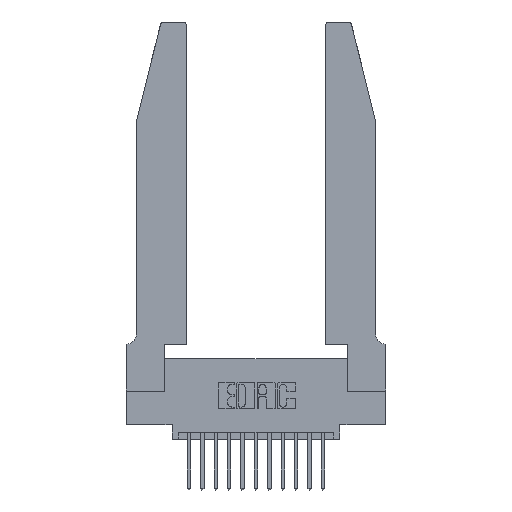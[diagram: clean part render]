
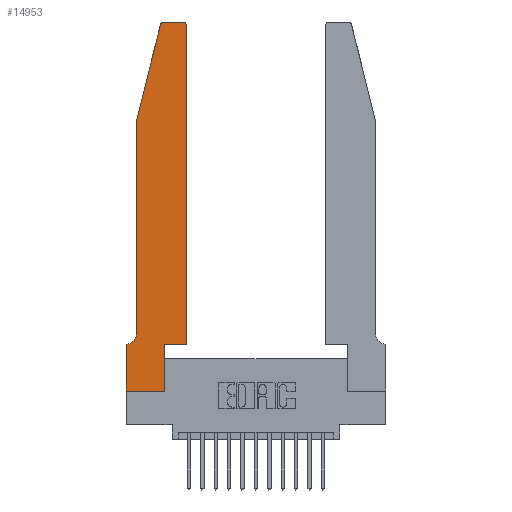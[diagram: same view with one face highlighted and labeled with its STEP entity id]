
A CAD part, top view. The second image highlights one B-rep face of the part: STEP entity #14953.
In plain terms, the highlighted planar face has unit normal (0, 0, 1).
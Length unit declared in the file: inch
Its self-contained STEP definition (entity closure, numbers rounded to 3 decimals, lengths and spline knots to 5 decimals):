
#7 = DIRECTION ( 'NONE',  ( 1., 0., 0. ) ) ;
#407 = ORIENTED_EDGE ( 'NONE', *, *, #14016, .T. ) ;
#790 = ORIENTED_EDGE ( 'NONE', *, *, #12398, .T. ) ;
#893 = VERTEX_POINT ( 'NONE', #1492 ) ;
#978 = DIRECTION ( 'NONE',  ( 1., 0., 0. ) ) ;
#989 = LINE ( 'NONE', #2405, #14650 ) ;
#1081 = CARTESIAN_POINT ( 'NONE',  ( 0., 0., 0.37 ) ) ;
#1184 = CARTESIAN_POINT ( 'NONE',  ( 0., 0., 0.37 ) ) ;
#1394 = CARTESIAN_POINT ( 'NONE',  ( 0.0755, 0.42, 0.37 ) ) ;
#1492 = CARTESIAN_POINT ( 'NONE',  ( 0.0755, 2., 0.37 ) ) ;
#1637 = CARTESIAN_POINT ( 'NONE',  ( 0.0755, 2., 0.37 ) ) ;
#1701 = CARTESIAN_POINT ( 'NONE',  ( 0.284, 2.75, 0.37 ) ) ;
#1876 = DIRECTION ( 'NONE',  ( 0., 0., 1. ) ) ;
#1938 = DIRECTION ( 'NONE',  ( 1., 0., 0. ) ) ;
#1939 = CARTESIAN_POINT ( 'NONE',  ( 0.2865, 0.35, 0.37 ) ) ;
#2405 = CARTESIAN_POINT ( 'NONE',  ( 0.4505, 0.35, 0.37 ) ) ;
#3024 = DIRECTION ( 'NONE',  ( 0., -1., 0. ) ) ;
#3386 = VECTOR ( 'NONE', #978, 39.37008 ) ;
#3550 = CARTESIAN_POINT ( 'NONE',  ( 0.4205, 2.72, 0.37 ) ) ;
#3747 = DIRECTION ( 'NONE',  ( -0.239, -0.971, 0. ) ) ;
#3759 = ORIENTED_EDGE ( 'NONE', *, *, #10830, .T. ) ;
#4178 = ORIENTED_EDGE ( 'NONE', *, *, #15427, .T. ) ;
#4341 = EDGE_CURVE ( 'NONE', #13516, #6120, #11697, .T. ) ;
#4379 = VERTEX_POINT ( 'NONE', #1939 ) ;
#4506 = VECTOR ( 'NONE', #4589, 39.37008 ) ;
#4589 = DIRECTION ( 'NONE',  ( -1., 0., 0. ) ) ;
#4610 = EDGE_CURVE ( 'NONE', #7141, #6379, #989, .T. ) ;
#4971 = DIRECTION ( 'NONE',  ( 1., 0., 0. ) ) ;
#5152 = EDGE_CURVE ( 'NONE', #8509, #10360, #8966, .T. ) ;
#5392 = DIRECTION ( 'NONE',  ( 0., -1., 0. ) ) ;
#5666 = VECTOR ( 'NONE', #13599, 39.37008 ) ;
#5779 = EDGE_CURVE ( 'NONE', #4379, #7141, #7053, .T. ) ;
#5937 = ORIENTED_EDGE ( 'NONE', *, *, #5152, .T. ) ;
#5962 = VERTEX_POINT ( 'NONE', #1394 ) ;
#6120 = VERTEX_POINT ( 'NONE', #1701 ) ;
#6379 = VERTEX_POINT ( 'NONE', #8123 ) ;
#6533 = CARTESIAN_POINT ( 'NONE',  ( 0.25487, 2.72718, 0.37 ) ) ;
#6922 = CIRCLE ( 'NONE', #6983, 0.07 ) ;
#6983 = AXIS2_PLACEMENT_3D ( 'NONE', #7587, #17018, #8947 ) ;
#7053 = LINE ( 'NONE', #10584, #3386 ) ;
#7141 = VERTEX_POINT ( 'NONE', #9866 ) ;
#7227 = VERTEX_POINT ( 'NONE', #10036 ) ;
#7254 = VECTOR ( 'NONE', #1938, 39.37008 ) ;
#7319 = LINE ( 'NONE', #8895, #10907 ) ;
#7341 = VECTOR ( 'NONE', #3024, 39.37008 ) ;
#7587 = CARTESIAN_POINT ( 'NONE',  ( 0.0055, 0.42, 0.37 ) ) ;
#7686 = LINE ( 'NONE', #14233, #7254 ) ;
#8092 = CIRCLE ( 'NONE', #12692, 0.03 ) ;
#8123 = CARTESIAN_POINT ( 'NONE',  ( 0.4505, 2.72, 0.37 ) ) ;
#8315 = DIRECTION ( 'NONE',  ( 0., 0., 1. ) ) ;
#8509 = VERTEX_POINT ( 'NONE', #8996 ) ;
#8895 = CARTESIAN_POINT ( 'NONE',  ( 0.2865, 0.35, 0.37 ) ) ;
#8947 = DIRECTION ( 'NONE',  ( -1., 0., 0. ) ) ;
#8966 = LINE ( 'NONE', #1184, #15686 ) ;
#8996 = CARTESIAN_POINT ( 'NONE',  ( 0., 0.35, 0.37 ) ) ;
#9045 = ORIENTED_EDGE ( 'NONE', *, *, #4610, .T. ) ;
#9215 = EDGE_CURVE ( 'NONE', #7227, #8509, #9261, .T. ) ;
#9261 = LINE ( 'NONE', #12238, #5666 ) ;
#9603 = EDGE_CURVE ( 'NONE', #5962, #7227, #6922, .T. ) ;
#9615 = EDGE_LOOP ( 'NONE', ( #13311, #4178, #3759, #12957, #10410, #14592, #5937, #10025, #790, #17001, #9045, #407 ) ) ;
#9866 = CARTESIAN_POINT ( 'NONE',  ( 0.4505, 0.35, 0.37 ) ) ;
#10025 = ORIENTED_EDGE ( 'NONE', *, *, #15005, .T. ) ;
#10036 = CARTESIAN_POINT ( 'NONE',  ( 0.0055, 0.35, 0.37 ) ) ;
#10040 = EDGE_CURVE ( 'NONE', #893, #5962, #14921, .T. ) ;
#10110 = PLANE ( 'NONE',  #10325 ) ;
#10325 = AXIS2_PLACEMENT_3D ( 'NONE', #14058, #1876, #11432 ) ;
#10360 = VERTEX_POINT ( 'NONE', #1081 ) ;
#10410 = ORIENTED_EDGE ( 'NONE', *, *, #9603, .T. ) ;
#10499 = CARTESIAN_POINT ( 'NONE',  ( 0.4205, 2.75, 0.37 ) ) ;
#10584 = CARTESIAN_POINT ( 'NONE',  ( 0.4505, 0.35, 0.37 ) ) ;
#10830 = EDGE_CURVE ( 'NONE', #13560, #893, #17017, .T. ) ;
#10907 = VECTOR ( 'NONE', #16962, 39.37008 ) ;
#11432 = DIRECTION ( 'NONE',  ( 1., 0., 0. ) ) ;
#11667 = FACE_OUTER_BOUND ( 'NONE', #9615, .T. ) ;
#11697 = LINE ( 'NONE', #15381, #4506 ) ;
#12012 = DIRECTION ( 'NONE',  ( 0., 1., 0. ) ) ;
#12227 = AXIS2_PLACEMENT_3D ( 'NONE', #3550, #13070, #4971 ) ;
#12238 = CARTESIAN_POINT ( 'NONE',  ( 0.0755, 0.35, 0.37 ) ) ;
#12398 = EDGE_CURVE ( 'NONE', #13905, #4379, #7319, .T. ) ;
#12692 = AXIS2_PLACEMENT_3D ( 'NONE', #16393, #8315, #7 ) ;
#12779 = CARTESIAN_POINT ( 'NONE',  ( 0.2865, 0., 0.37 ) ) ;
#12957 = ORIENTED_EDGE ( 'NONE', *, *, #10040, .T. ) ;
#13070 = DIRECTION ( 'NONE',  ( 0., 0., 1. ) ) ;
#13311 = ORIENTED_EDGE ( 'NONE', *, *, #4341, .T. ) ;
#13424 = VECTOR ( 'NONE', #3747, 39.37008 ) ;
#13516 = VERTEX_POINT ( 'NONE', #10499 ) ;
#13560 = VERTEX_POINT ( 'NONE', #6533 ) ;
#13599 = DIRECTION ( 'NONE',  ( -1., 0., 0. ) ) ;
#13905 = VERTEX_POINT ( 'NONE', #12779 ) ;
#14016 = EDGE_CURVE ( 'NONE', #6379, #13516, #15294, .T. ) ;
#14058 = CARTESIAN_POINT ( 'NONE',  ( 0., 0.35, 0.37 ) ) ;
#14233 = CARTESIAN_POINT ( 'NONE',  ( 0., 0., 0.37 ) ) ;
#14592 = ORIENTED_EDGE ( 'NONE', *, *, #9215, .T. ) ;
#14650 = VECTOR ( 'NONE', #12012, 39.37008 ) ;
#14921 = LINE ( 'NONE', #1637, #7341 ) ;
#14953 = ADVANCED_FACE ( 'NONE', ( #11667 ), #10110, .T. ) ;
#15005 = EDGE_CURVE ( 'NONE', #10360, #13905, #7686, .T. ) ;
#15294 = CIRCLE ( 'NONE', #12227, 0.03 ) ;
#15381 = CARTESIAN_POINT ( 'NONE',  ( 0.2605, 2.75, 0.37 ) ) ;
#15427 = EDGE_CURVE ( 'NONE', #6120, #13560, #8092, .T. ) ;
#15686 = VECTOR ( 'NONE', #5392, 39.37008 ) ;
#16393 = CARTESIAN_POINT ( 'NONE',  ( 0.284, 2.72, 0.37 ) ) ;
#16962 = DIRECTION ( 'NONE',  ( 0., 1., 0. ) ) ;
#17001 = ORIENTED_EDGE ( 'NONE', *, *, #5779, .T. ) ;
#17017 = LINE ( 'NONE', #17261, #13424 ) ;
#17018 = DIRECTION ( 'NONE',  ( 0., 0., -1. ) ) ;
#17261 = CARTESIAN_POINT ( 'NONE',  ( 0.0755, 2., 0.37 ) ) ;
